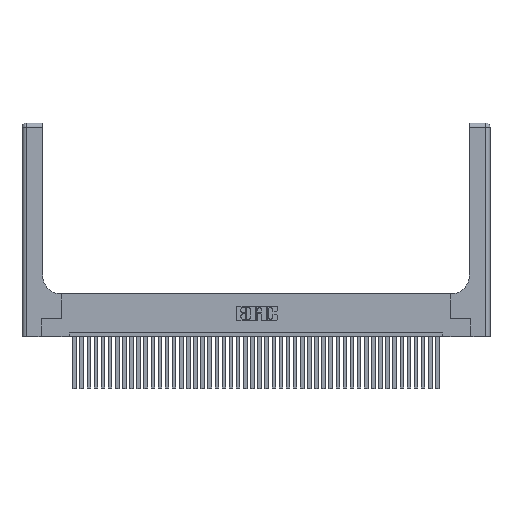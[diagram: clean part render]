
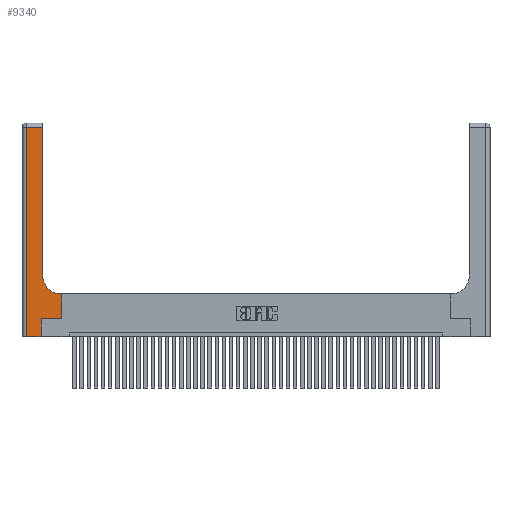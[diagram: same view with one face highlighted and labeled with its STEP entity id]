
A CAD part, top view. The second image highlights one B-rep face of the part: STEP entity #9340.
In plain terms, the highlighted planar face has unit normal (0, 0, 1).
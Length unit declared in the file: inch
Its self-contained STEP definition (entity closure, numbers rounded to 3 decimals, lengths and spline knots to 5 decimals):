
#438 = CARTESIAN_POINT ( 'NONE',  ( 0.2915, 0.6, 0.37 ) ) ;
#839 = ORIENTED_EDGE ( 'NONE', *, *, #5412, .T. ) ;
#1358 = ORIENTED_EDGE ( 'NONE', *, *, #31003, .T. ) ;
#1414 = CARTESIAN_POINT ( 'NONE',  ( 0.269, 0., 0.37 ) ) ;
#2074 = EDGE_CURVE ( 'NONE', #15745, #2823, #17103, .T. ) ;
#2823 = VERTEX_POINT ( 'NONE', #1414 ) ;
#3328 = DIRECTION ( 'NONE',  ( -1., 0., 0. ) ) ;
#5013 = DIRECTION ( 'NONE',  ( -1., 0., 0. ) ) ;
#5119 = VECTOR ( 'NONE', #3328, 39.37008 ) ;
#5355 = VERTEX_POINT ( 'NONE', #34684 ) ;
#5412 = EDGE_CURVE ( 'NONE', #42647, #21173, #39426, .T. ) ;
#5881 = CARTESIAN_POINT ( 'NONE',  ( 0.5585, 0.6, 0.37 ) ) ;
#7039 = CARTESIAN_POINT ( 'NONE',  ( 0.06, 0., 0.37 ) ) ;
#7723 = CARTESIAN_POINT ( 'NONE',  ( 0.5415, 0.6, 0.37 ) ) ;
#8499 = CARTESIAN_POINT ( 'NONE',  ( 0.06, 3., 0.37 ) ) ;
#8629 = DIRECTION ( 'NONE',  ( 0., 0., -1. ) ) ;
#8712 = AXIS2_PLACEMENT_3D ( 'NONE', #31871, #8629, #28956 ) ;
#9253 = ORIENTED_EDGE ( 'NONE', *, *, #41506, .T. ) ;
#9340 = ADVANCED_FACE ( 'NONE', ( #21006 ), #22256, .F. ) ;
#9538 = AXIS2_PLACEMENT_3D ( 'NONE', #12704, #22396, #25721 ) ;
#10268 = VECTOR ( 'NONE', #5013, 39.37008 ) ;
#10352 = CIRCLE ( 'NONE', #8712, 0.25 ) ;
#10400 = ORIENTED_EDGE ( 'NONE', *, *, #14230, .T. ) ;
#11151 = DIRECTION ( 'NONE',  ( 0., 1., 0. ) ) ;
#11896 = ORIENTED_EDGE ( 'NONE', *, *, #31644, .T. ) ;
#12366 = LINE ( 'NONE', #33231, #17505 ) ;
#12704 = CARTESIAN_POINT ( 'NONE',  ( 0., 3., 0.37 ) ) ;
#12821 = LINE ( 'NONE', #438, #5119 ) ;
#13020 = VECTOR ( 'NONE', #34540, 39.37008 ) ;
#13913 = CARTESIAN_POINT ( 'NONE',  ( 0., 2.94, 0.37 ) ) ;
#13929 = VECTOR ( 'NONE', #24187, 39.37008 ) ;
#14230 = EDGE_CURVE ( 'NONE', #2823, #5355, #24516, .T. ) ;
#15219 = EDGE_LOOP ( 'NONE', ( #839, #36576, #17214, #18277, #10400, #9253, #1358, #11896, #40689 ) ) ;
#15712 = VERTEX_POINT ( 'NONE', #36512 ) ;
#15745 = VERTEX_POINT ( 'NONE', #7039 ) ;
#15895 = CARTESIAN_POINT ( 'NONE',  ( 0.2915, 0.85, 0.37 ) ) ;
#16734 = VECTOR ( 'NONE', #11151, 39.37008 ) ;
#17103 = LINE ( 'NONE', #40616, #39922 ) ;
#17214 = ORIENTED_EDGE ( 'NONE', *, *, #28207, .T. ) ;
#17505 = VECTOR ( 'NONE', #29463, 39.37008 ) ;
#18277 = ORIENTED_EDGE ( 'NONE', *, *, #2074, .T. ) ;
#18553 = LINE ( 'NONE', #8499, #40321 ) ;
#19435 = EDGE_CURVE ( 'NONE', #33764, #42647, #10352, .T. ) ;
#19447 = VERTEX_POINT ( 'NONE', #5881 ) ;
#21006 = FACE_OUTER_BOUND ( 'NONE', #15219, .T. ) ;
#21173 = VERTEX_POINT ( 'NONE', #22294 ) ;
#22256 = PLANE ( 'NONE',  #9538 ) ;
#22294 = CARTESIAN_POINT ( 'NONE',  ( 0.2915, 2.94, 0.37 ) ) ;
#22396 = DIRECTION ( 'NONE',  ( 0., 0., -1. ) ) ;
#24187 = DIRECTION ( 'NONE',  ( 1., 0., 0. ) ) ;
#24516 = LINE ( 'NONE', #27878, #16734 ) ;
#25721 = DIRECTION ( 'NONE',  ( -1., 0., 0. ) ) ;
#27490 = CARTESIAN_POINT ( 'NONE',  ( 0.269, 0.25, 0.37 ) ) ;
#27878 = CARTESIAN_POINT ( 'NONE',  ( 0.269, 0., 0.37 ) ) ;
#28207 = EDGE_CURVE ( 'NONE', #15712, #15745, #18553, .T. ) ;
#28586 = EDGE_CURVE ( 'NONE', #21173, #15712, #36655, .T. ) ;
#28956 = DIRECTION ( 'NONE',  ( 1., 0., 0. ) ) ;
#29463 = DIRECTION ( 'NONE',  ( 0., 1., 0. ) ) ;
#29960 = LINE ( 'NONE', #27490, #13929 ) ;
#31003 = EDGE_CURVE ( 'NONE', #38628, #19447, #12366, .T. ) ;
#31644 = EDGE_CURVE ( 'NONE', #19447, #33764, #12821, .T. ) ;
#31871 = CARTESIAN_POINT ( 'NONE',  ( 0.5415, 0.85, 0.37 ) ) ;
#33231 = CARTESIAN_POINT ( 'NONE',  ( 0.5585, 0.25, 0.37 ) ) ;
#33764 = VERTEX_POINT ( 'NONE', #7723 ) ;
#33805 = DIRECTION ( 'NONE',  ( 1., 0., 0. ) ) ;
#34540 = DIRECTION ( 'NONE',  ( 0., 1., 0. ) ) ;
#34684 = CARTESIAN_POINT ( 'NONE',  ( 0.269, 0.25, 0.37 ) ) ;
#36512 = CARTESIAN_POINT ( 'NONE',  ( 0.06, 2.94, 0.37 ) ) ;
#36576 = ORIENTED_EDGE ( 'NONE', *, *, #28586, .T. ) ;
#36655 = LINE ( 'NONE', #13913, #10268 ) ;
#37461 = CARTESIAN_POINT ( 'NONE',  ( 0.2915, 3., 0.37 ) ) ;
#38288 = DIRECTION ( 'NONE',  ( 0., -1., 0. ) ) ;
#38628 = VERTEX_POINT ( 'NONE', #40225 ) ;
#39426 = LINE ( 'NONE', #37461, #13020 ) ;
#39922 = VECTOR ( 'NONE', #33805, 39.37008 ) ;
#40225 = CARTESIAN_POINT ( 'NONE',  ( 0.5585, 0.25, 0.37 ) ) ;
#40321 = VECTOR ( 'NONE', #38288, 39.37008 ) ;
#40616 = CARTESIAN_POINT ( 'NONE',  ( 0., 0., 0.37 ) ) ;
#40689 = ORIENTED_EDGE ( 'NONE', *, *, #19435, .T. ) ;
#41506 = EDGE_CURVE ( 'NONE', #5355, #38628, #29960, .T. ) ;
#42647 = VERTEX_POINT ( 'NONE', #15895 ) ;
